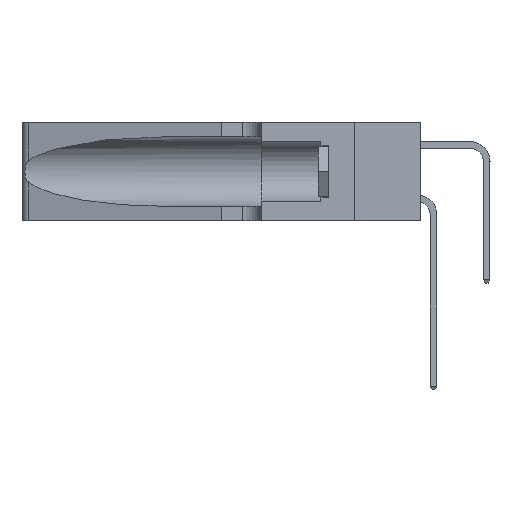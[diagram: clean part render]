
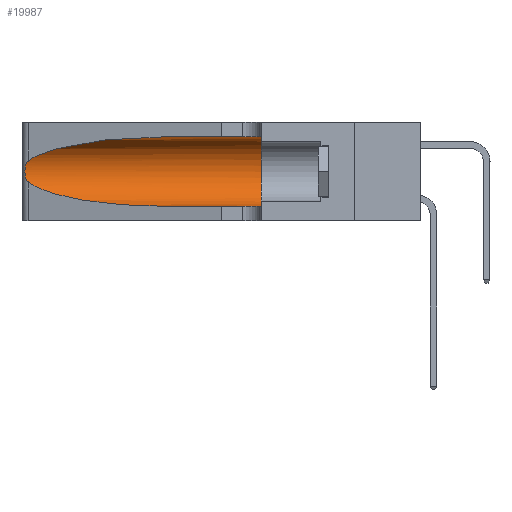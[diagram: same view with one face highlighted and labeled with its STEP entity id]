
A CAD part, left-side view. The second image highlights one B-rep face of the part: STEP entity #19987.
In plain terms, the highlighted cylindrical face has radius 3.308 mm (diameter 6.617 mm), a partial arc.
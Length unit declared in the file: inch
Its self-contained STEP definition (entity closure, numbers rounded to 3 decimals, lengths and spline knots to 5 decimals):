
#446 = EDGE_CURVE ( 'NONE', #794, #17453, #4407, .T. ) ;
#794 = VERTEX_POINT ( 'NONE', #9221 ) ;
#904 = CARTESIAN_POINT ( 'NONE',  ( 0.26018, 1.23835, 0.19895 ) ) ;
#954 = DIRECTION ( 'NONE',  ( 0., -1., 0. ) ) ;
#1188 = CARTESIAN_POINT ( 'NONE',  ( 0.26075, 1.23896, 0.19203 ) ) ;
#1422 = CYLINDRICAL_SURFACE ( 'NONE', #21152, 0.13025 ) ;
#2227 = CARTESIAN_POINT ( 'NONE',  ( 0.1305, 1.61858, 0.185 ) ) ;
#2644 = CARTESIAN_POINT ( 'NONE',  ( 0.25487, 1.22718, 0.14631 ) ) ;
#2908 = B_SPLINE_CURVE_WITH_KNOTS ( 'NONE', 3,
 ( #26646, #26746, #13647, #5512, #9906, #904, #1188, #25080, #14138, #20503, #24894, #12007, #18438, #25174 ),
 .UNSPECIFIED., .F., .F.,
 ( 4, 2, 2, 2, 2, 2, 4 ),
 ( 0., 0.00027, 0.00053, 0.00107, 0.0016, 0.00187, 0.00214 ),
 .UNSPECIFIED. ) ;
#3476 = VERTEX_POINT ( 'NONE', #10063 ) ;
#4407 = LINE ( 'NONE', #18599, #23907 ) ;
#4801 = EDGE_LOOP ( 'NONE', ( #16864, #5494, #11023, #20585, #22189, #24081 ) ) ;
#5403 = EDGE_CURVE ( 'NONE', #794, #17076, #27807, .T. ) ;
#5494 = ORIENTED_EDGE ( 'NONE', *, *, #12363, .T. ) ;
#5512 = CARTESIAN_POINT ( 'NONE',  ( 0.25787, 1.23484, 0.2124 ) ) ;
#5560 = CIRCLE ( 'NONE', #20600, 0.13025 ) ;
#6648 = CARTESIAN_POINT ( 'NONE',  ( 0.25487, 1.22718, 0.22369 ) ) ;
#6989 = CARTESIAN_POINT ( 'NONE',  ( 0.1305, 0.72297, 0.05475 ) ) ;
#7784 = DIRECTION ( 'NONE',  ( 0., -1., 0. ) ) ;
#7886 = VERTEX_POINT ( 'NONE', #10154 ) ;
#8971 = DIRECTION ( 'NONE',  ( 0., -1., 0. ) ) ;
#9163 = LINE ( 'NONE', #22791, #25500 ) ;
#9221 = CARTESIAN_POINT ( 'NONE',  ( 0.1305, 0.72297, 0.31525 ) ) ;
#9730 = CARTESIAN_POINT ( 'NONE',  ( 0.25487, 1.22718, 0.22369 ) ) ;
#9906 = CARTESIAN_POINT ( 'NONE',  ( 0.25854, 1.2359, 0.20912 ) ) ;
#10063 = CARTESIAN_POINT ( 'NONE',  ( 0.1305, 0.72297, 0.05475 ) ) ;
#10154 = CARTESIAN_POINT ( 'NONE',  ( 0.25487, 1.22718, 0.14631 ) ) ;
#11023 = ORIENTED_EDGE ( 'NONE', *, *, #26678, .T. ) ;
#11419 = CARTESIAN_POINT ( 'NONE',  ( 0.1305, 0.35, 0.31525 ) ) ;
#11845 = VERTEX_POINT ( 'NONE', #24230 ) ;
#12007 = CARTESIAN_POINT ( 'NONE',  ( 0.25639, 1.23186, 0.15144 ) ) ;
#12363 = EDGE_CURVE ( 'NONE', #17076, #7886, #2908, .T. ) ;
#13647 = CARTESIAN_POINT ( 'NONE',  ( 0.25639, 1.23184, 0.21858 ) ) ;
#14138 = CARTESIAN_POINT ( 'NONE',  ( 0.26017, 1.23833, 0.17102 ) ) ;
#14469 = FACE_OUTER_BOUND ( 'NONE', #4801, .T. ) ;
#15521 = CARTESIAN_POINT ( 'NONE',  ( 0.2373, 1.15595, 0.28018 ) ) ;
#16864 = ORIENTED_EDGE ( 'NONE', *, *, #5403, .T. ) ;
#17076 = VERTEX_POINT ( 'NONE', #9730 ) ;
#17353 = CARTESIAN_POINT ( 'NONE',  ( 0.18966, 0.96281, 0.31525 ) ) ;
#17453 = VERTEX_POINT ( 'NONE', #11419 ) ;
#17783 = CARTESIAN_POINT ( 'NONE',  ( 0.18966, 0.96281, 0.05475 ) ) ;
#18438 = CARTESIAN_POINT ( 'NONE',  ( 0.25555, 1.22993, 0.14849 ) ) ;
#18599 = CARTESIAN_POINT ( 'NONE',  ( 0.1305, 1.61858, 0.31525 ) ) ;
#19573 = DIRECTION ( 'NONE',  ( 0., 0., -1. ) ) ;
#19887 = EDGE_CURVE ( 'NONE', #17453, #11845, #5560, .T. ) ;
#19987 = ADVANCED_FACE ( 'NONE', ( #14469 ), #1422, .F. ) ;
#20503 = CARTESIAN_POINT ( 'NONE',  ( 0.25856, 1.23593, 0.16098 ) ) ;
#20585 = ORIENTED_EDGE ( 'NONE', *, *, #24801, .T. ) ;
#20600 = AXIS2_PLACEMENT_3D ( 'NONE', #24986, #20791, #23008 ) ;
#20791 = DIRECTION ( 'NONE',  ( 0., 1., 0. ) ) ;
#21152 = AXIS2_PLACEMENT_3D ( 'NONE', #2227, #8971, #19573 ) ;
#22122 = CARTESIAN_POINT ( 'NONE',  ( 0.1305, 0.72297, 0.31525 ) ) ;
#22189 = ORIENTED_EDGE ( 'NONE', *, *, #19887, .F. ) ;
#22791 = CARTESIAN_POINT ( 'NONE',  ( 0.1305, 1.61858, 0.05475 ) ) ;
#23008 = DIRECTION ( 'NONE',  ( 0., 0., 1. ) ) ;
#23241 =( BOUNDED_CURVE ( )  B_SPLINE_CURVE ( 3, ( #2644, #24163, #17783, #6989 ),
 .UNSPECIFIED., .F., .F. ) 
 B_SPLINE_CURVE_WITH_KNOTS ( ( 4, 4 ),
 ( 3.44316, 4.71239 ),
 .UNSPECIFIED. ) 
 CURVE ( )  GEOMETRIC_REPRESENTATION_ITEM ( )  RATIONAL_B_SPLINE_CURVE ( ( 1., 0.87, 0.87, 1. ) ) 
 REPRESENTATION_ITEM ( '' )  );
#23907 = VECTOR ( 'NONE', #7784, 39.37008 ) ;
#24081 = ORIENTED_EDGE ( 'NONE', *, *, #446, .F. ) ;
#24163 = CARTESIAN_POINT ( 'NONE',  ( 0.2373, 1.15595, 0.08982 ) ) ;
#24230 = CARTESIAN_POINT ( 'NONE',  ( 0.1305, 0.35, 0.05475 ) ) ;
#24801 = EDGE_CURVE ( 'NONE', #3476, #11845, #9163, .T. ) ;
#24894 = CARTESIAN_POINT ( 'NONE',  ( 0.25789, 1.23486, 0.15765 ) ) ;
#24986 = CARTESIAN_POINT ( 'NONE',  ( 0.1305, 0.35, 0.185 ) ) ;
#25080 = CARTESIAN_POINT ( 'NONE',  ( 0.26075, 1.23896, 0.178 ) ) ;
#25174 = CARTESIAN_POINT ( 'NONE',  ( 0.25487, 1.22718, 0.14631 ) ) ;
#25500 = VECTOR ( 'NONE', #954, 39.37008 ) ;
#26646 = CARTESIAN_POINT ( 'NONE',  ( 0.25487, 1.22718, 0.22369 ) ) ;
#26678 = EDGE_CURVE ( 'NONE', #7886, #3476, #23241, .T. ) ;
#26746 = CARTESIAN_POINT ( 'NONE',  ( 0.25555, 1.22994, 0.2215 ) ) ;
#27807 =( BOUNDED_CURVE ( )  B_SPLINE_CURVE ( 3, ( #22122, #17353, #15521, #6648 ),
 .UNSPECIFIED., .F., .F. ) 
 B_SPLINE_CURVE_WITH_KNOTS ( ( 4, 4 ),
 ( 1.5708, 2.84003 ),
 .UNSPECIFIED. ) 
 CURVE ( )  GEOMETRIC_REPRESENTATION_ITEM ( )  RATIONAL_B_SPLINE_CURVE ( ( 1., 0.87, 0.87, 1. ) ) 
 REPRESENTATION_ITEM ( '' )  );
